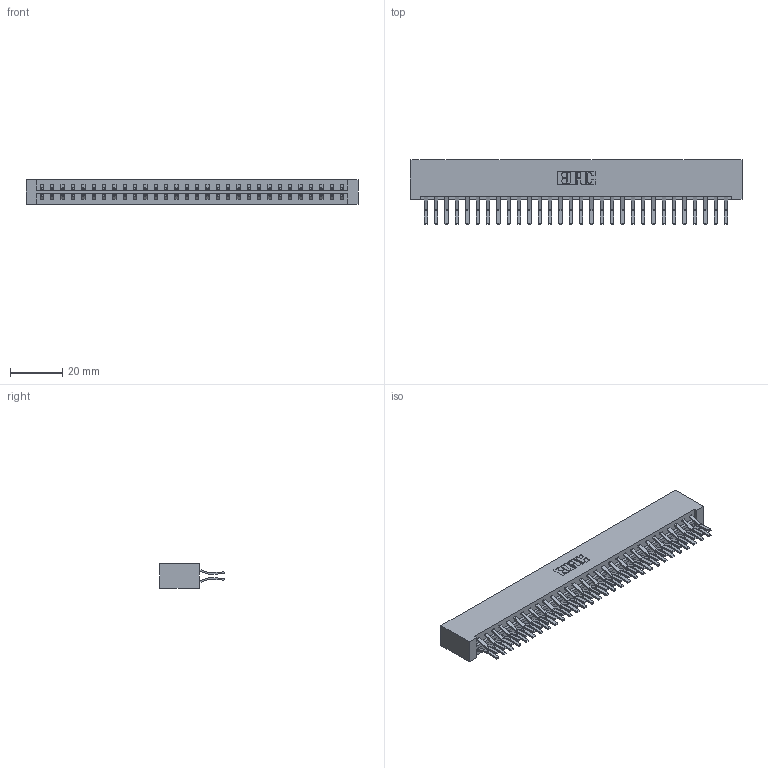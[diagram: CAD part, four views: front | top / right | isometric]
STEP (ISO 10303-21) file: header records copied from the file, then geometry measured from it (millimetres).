
FILE_DESCRIPTION (( 'STEP AP203' ), '1' );
FILE_NAME ('333-060-560-201.STEP', '2018-08-04T07:52:43', ( '' ), ( '' ), 'SwSTEP 2.0', 'SolidWorks 2016', '' );
FILE_SCHEMA (( 'CONFIG_CONTROL_DESIGN' ));
Length unit declared in the file: inch
Products named in the file (3): 333 Part_Lugless; 345-292-001_560 Tail; 333-060-560-201
Assembly tree (61 placements, depth 2):
  333-060-560-201
    333 Part_Lugless
    345-292-001_560 Tail  x60
Bounding box: 127.13 x 24.78 x 9.4 mm (x, y, z)
Volume: 13892.2 mm3; surface area: 17441.4 mm2
Topology: 61 solids, 61 shells, 3346 faces, 9947 edges, 6550 vertices
Faces by surface type: plane 2226, cylinder 1120
Entity records: 20663 total; most frequent: CARTESIAN_POINT 3438, ORIENTED_EDGE 3374, DIRECTION 2955, EDGE_CURVE 1687, LINE 1563, VECTOR 1563, VERTEX_POINT 1122, AXIS2_PLACEMENT_3D 696
